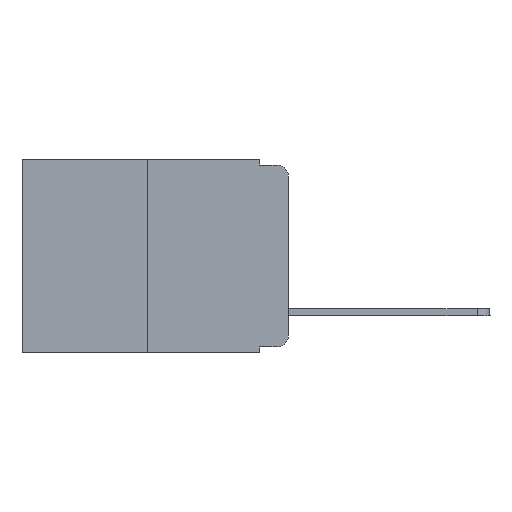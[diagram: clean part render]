
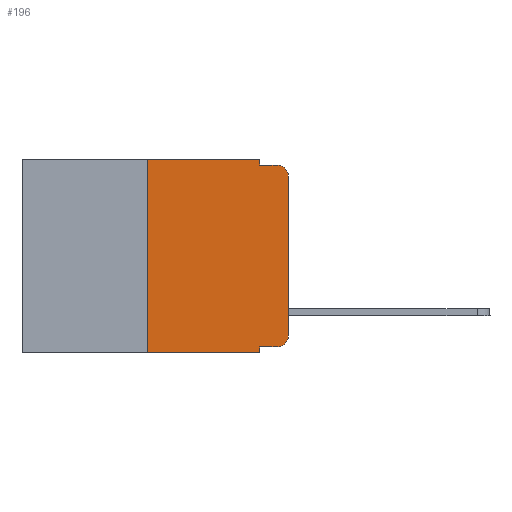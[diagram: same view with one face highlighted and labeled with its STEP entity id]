
A CAD part, left-side view. The second image highlights one B-rep face of the part: STEP entity #196.
In plain terms, the highlighted planar face has unit normal (-1, 0, 0).
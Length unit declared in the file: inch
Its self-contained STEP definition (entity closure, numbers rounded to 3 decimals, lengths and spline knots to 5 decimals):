
#196 = ADVANCED_FACE ( 'NONE', ( #10968 ), #8324, .F. ) ;
#329 = DIRECTION ( 'NONE',  ( 0., 0., -1. ) ) ;
#580 = DIRECTION ( 'NONE',  ( 0., -1., 0. ) ) ;
#683 = VECTOR ( 'NONE', #7126, 39.37008 ) ;
#813 = VECTOR ( 'NONE', #9807, 39.37008 ) ;
#834 = VERTEX_POINT ( 'NONE', #8931 ) ;
#1046 = EDGE_CURVE ( 'NONE', #1564, #2956, #2178, .T. ) ;
#1210 = CARTESIAN_POINT ( 'NONE',  ( 0., 0.473, -0.343 ) ) ;
#1269 = VERTEX_POINT ( 'NONE', #6140 ) ;
#1358 = DIRECTION ( 'NONE',  ( 0., -1., 0. ) ) ;
#1564 = VERTEX_POINT ( 'NONE', #7013 ) ;
#1657 = ORIENTED_EDGE ( 'NONE', *, *, #7932, .F. ) ;
#1785 = DIRECTION ( 'NONE',  ( 0., 0., -1. ) ) ;
#1803 = ORIENTED_EDGE ( 'NONE', *, *, #7128, .T. ) ;
#1838 = VECTOR ( 'NONE', #4282, 39.37008 ) ;
#1854 = VERTEX_POINT ( 'NONE', #10841 ) ;
#1922 = LINE ( 'NONE', #3879, #10700 ) ;
#2020 = CARTESIAN_POINT ( 'NONE',  ( 0., 0.051, 0. ) ) ;
#2178 = LINE ( 'NONE', #2020, #7097 ) ;
#2324 = VERTEX_POINT ( 'NONE', #3116 ) ;
#2331 = VECTOR ( 'NONE', #10637, 39.37008 ) ;
#2422 = ORIENTED_EDGE ( 'NONE', *, *, #3626, .T. ) ;
#2444 = VERTEX_POINT ( 'NONE', #5887 ) ;
#2662 = LINE ( 'NONE', #1210, #683 ) ;
#2720 = DIRECTION ( 'NONE',  ( -1., 0., 0. ) ) ;
#2846 = ORIENTED_EDGE ( 'NONE', *, *, #1046, .F. ) ;
#2956 = VERTEX_POINT ( 'NONE', #9351 ) ;
#3004 = ORIENTED_EDGE ( 'NONE', *, *, #6113, .F. ) ;
#3088 = DIRECTION ( 'NONE',  ( -1., 0., 0. ) ) ;
#3116 = CARTESIAN_POINT ( 'NONE',  ( 0., 0., -0.313 ) ) ;
#3244 = CARTESIAN_POINT ( 'NONE',  ( 0., 0.02, -0.03 ) ) ;
#3626 = EDGE_CURVE ( 'NONE', #5083, #2324, #4320, .T. ) ;
#3629 = CARTESIAN_POINT ( 'NONE',  ( 0., 0.051, 0. ) ) ;
#3674 = ORIENTED_EDGE ( 'NONE', *, *, #5375, .F. ) ;
#3701 = CARTESIAN_POINT ( 'NONE',  ( 0., 0., 0. ) ) ;
#3833 = EDGE_CURVE ( 'NONE', #2444, #1854, #4592, .T. ) ;
#3879 = CARTESIAN_POINT ( 'NONE',  ( 0., 0.051, -0.01 ) ) ;
#4047 = CARTESIAN_POINT ( 'NONE',  ( 0., 0.02, -0.333 ) ) ;
#4095 = CARTESIAN_POINT ( 'NONE',  ( 0., 0.473, 0. ) ) ;
#4282 = DIRECTION ( 'NONE',  ( 0., -1., 0. ) ) ;
#4320 = CIRCLE ( 'NONE', #7369, 0.02 ) ;
#4592 = LINE ( 'NONE', #4643, #2331 ) ;
#4643 = CARTESIAN_POINT ( 'NONE',  ( 0., 0.25, 0. ) ) ;
#4895 = EDGE_CURVE ( 'NONE', #2444, #1269, #2662, .T. ) ;
#5083 = VERTEX_POINT ( 'NONE', #4047 ) ;
#5375 = EDGE_CURVE ( 'NONE', #834, #1269, #7041, .T. ) ;
#5424 = VECTOR ( 'NONE', #1358, 39.37008 ) ;
#5651 = EDGE_LOOP ( 'NONE', ( #10453, #10053, #1657, #2846, #3004, #6335, #5884, #3674, #1803, #2422 ) ) ;
#5838 = CIRCLE ( 'NONE', #10208, 0.02 ) ;
#5884 = ORIENTED_EDGE ( 'NONE', *, *, #4895, .T. ) ;
#5887 = CARTESIAN_POINT ( 'NONE',  ( 0., 0.25, -0.343 ) ) ;
#5970 = LINE ( 'NONE', #8418, #1838 ) ;
#6006 = EDGE_CURVE ( 'NONE', #10185, #9295, #5838, .T. ) ;
#6113 = EDGE_CURVE ( 'NONE', #1854, #1564, #5970, .T. ) ;
#6140 = CARTESIAN_POINT ( 'NONE',  ( 0., 0.051, -0.343 ) ) ;
#6335 = ORIENTED_EDGE ( 'NONE', *, *, #3833, .F. ) ;
#6399 = EDGE_CURVE ( 'NONE', #2324, #10185, #9012, .T. ) ;
#6635 = DIRECTION ( 'NONE',  ( 0., 0., -1. ) ) ;
#6947 = CARTESIAN_POINT ( 'NONE',  ( 0., 0.02, -0.313 ) ) ;
#7013 = CARTESIAN_POINT ( 'NONE',  ( 0., 0.051, 0. ) ) ;
#7041 = LINE ( 'NONE', #3629, #813 ) ;
#7097 = VECTOR ( 'NONE', #329, 39.37008 ) ;
#7126 = DIRECTION ( 'NONE',  ( 0., -1., 0. ) ) ;
#7128 = EDGE_CURVE ( 'NONE', #834, #5083, #7683, .T. ) ;
#7284 = CARTESIAN_POINT ( 'NONE',  ( 0., 0.051, -0.333 ) ) ;
#7369 = AXIS2_PLACEMENT_3D ( 'NONE', #6947, #2720, #1785 ) ;
#7683 = LINE ( 'NONE', #7284, #5424 ) ;
#7898 = DIRECTION ( 'NONE',  ( 0., 0., 1. ) ) ;
#7932 = EDGE_CURVE ( 'NONE', #2956, #9295, #1922, .T. ) ;
#8066 = AXIS2_PLACEMENT_3D ( 'NONE', #4095, #10037, #6635 ) ;
#8324 = PLANE ( 'NONE',  #8066 ) ;
#8418 = CARTESIAN_POINT ( 'NONE',  ( 0., 0.473, 0. ) ) ;
#8419 = CARTESIAN_POINT ( 'NONE',  ( 0., 0., -0.03 ) ) ;
#8931 = CARTESIAN_POINT ( 'NONE',  ( 0., 0.051, -0.333 ) ) ;
#9012 = LINE ( 'NONE', #3701, #10213 ) ;
#9199 = DIRECTION ( 'NONE',  ( 0., 0., -1. ) ) ;
#9295 = VERTEX_POINT ( 'NONE', #10945 ) ;
#9351 = CARTESIAN_POINT ( 'NONE',  ( 0., 0.051, -0.01 ) ) ;
#9807 = DIRECTION ( 'NONE',  ( 0., 0., -1. ) ) ;
#10037 = DIRECTION ( 'NONE',  ( 1., 0., 0. ) ) ;
#10053 = ORIENTED_EDGE ( 'NONE', *, *, #6006, .T. ) ;
#10185 = VERTEX_POINT ( 'NONE', #8419 ) ;
#10208 = AXIS2_PLACEMENT_3D ( 'NONE', #3244, #3088, #9199 ) ;
#10213 = VECTOR ( 'NONE', #7898, 39.37008 ) ;
#10453 = ORIENTED_EDGE ( 'NONE', *, *, #6399, .T. ) ;
#10637 = DIRECTION ( 'NONE',  ( 0., 0., 1. ) ) ;
#10700 = VECTOR ( 'NONE', #580, 39.37008 ) ;
#10841 = CARTESIAN_POINT ( 'NONE',  ( 0., 0.25, 0. ) ) ;
#10945 = CARTESIAN_POINT ( 'NONE',  ( 0., 0.02, -0.01 ) ) ;
#10968 = FACE_OUTER_BOUND ( 'NONE', #5651, .T. ) ;
